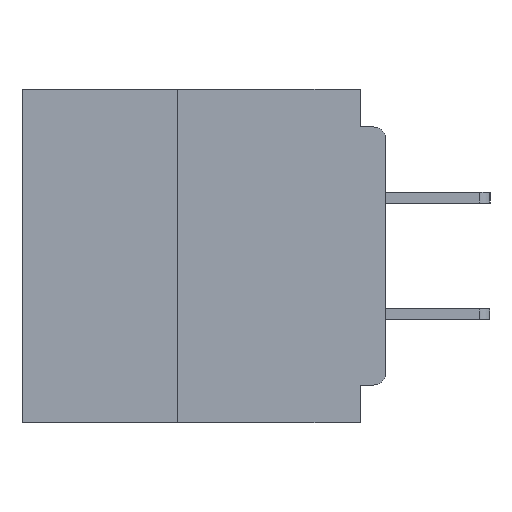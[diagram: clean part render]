
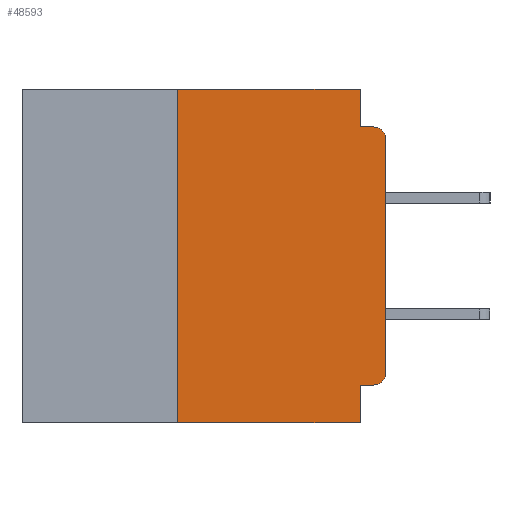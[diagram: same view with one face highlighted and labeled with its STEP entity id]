
A CAD part, left-side view. The second image highlights one B-rep face of the part: STEP entity #48593.
In plain terms, the highlighted planar face has unit normal (-1, 0, 0).
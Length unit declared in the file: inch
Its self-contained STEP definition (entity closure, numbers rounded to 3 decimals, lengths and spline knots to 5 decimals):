
#178 = CARTESIAN_POINT ( 'NONE',  ( 0., 0.031, -0.4 ) ) ;
#2122 = CARTESIAN_POINT ( 'NONE',  ( 0., 0., -0.355 ) ) ;
#2976 = EDGE_CURVE ( 'NONE', #23231, #23133, #15568, .T. ) ;
#4023 = DIRECTION ( 'NONE',  ( 0., 0., -1. ) ) ;
#4742 = CARTESIAN_POINT ( 'NONE',  ( 0., 0.015, -0.355 ) ) ;
#6168 = CARTESIAN_POINT ( 'NONE',  ( 0., 0.031, -0.4 ) ) ;
#6310 = AXIS2_PLACEMENT_3D ( 'NONE', #19619, #46124, #23431 ) ;
#6483 = ORIENTED_EDGE ( 'NONE', *, *, #15444, .F. ) ;
#6874 = DIRECTION ( 'NONE',  ( 0., 0., 1. ) ) ;
#7160 = EDGE_CURVE ( 'NONE', #12666, #23231, #46648, .T. ) ;
#7787 = CARTESIAN_POINT ( 'NONE',  ( 0., 0., -0.045 ) ) ;
#8104 = EDGE_CURVE ( 'NONE', #19189, #9702, #42371, .T. ) ;
#9702 = VERTEX_POINT ( 'NONE', #12455 ) ;
#9875 = LINE ( 'NONE', #178, #12223 ) ;
#12223 = VECTOR ( 'NONE', #4023, 39.37008 ) ;
#12455 = CARTESIAN_POINT ( 'NONE',  ( 0., 0.031, -0.355 ) ) ;
#12594 = DIRECTION ( 'NONE',  ( 0., 0., -1. ) ) ;
#12666 = VERTEX_POINT ( 'NONE', #37422 ) ;
#12769 = EDGE_CURVE ( 'NONE', #9702, #44273, #9875, .T. ) ;
#13081 = VECTOR ( 'NONE', #38442, 39.37008 ) ;
#14164 = ORIENTED_EDGE ( 'NONE', *, *, #8104, .F. ) ;
#14727 = ORIENTED_EDGE ( 'NONE', *, *, #15273, .T. ) ;
#15144 = VECTOR ( 'NONE', #35026, 39.37008 ) ;
#15273 = EDGE_CURVE ( 'NONE', #48046, #44273, #24328, .T. ) ;
#15444 = EDGE_CURVE ( 'NONE', #29797, #28308, #35060, .T. ) ;
#15518 = EDGE_LOOP ( 'NONE', ( #47272, #30776, #42019, #35539, #6483, #49037, #14727, #44966, #14164, #15943 ) ) ;
#15568 = CIRCLE ( 'NONE', #18995, 0.015 ) ;
#15777 = CARTESIAN_POINT ( 'NONE',  ( 0., 0.031, 0. ) ) ;
#15943 = ORIENTED_EDGE ( 'NONE', *, *, #42050, .T. ) ;
#16989 = CARTESIAN_POINT ( 'NONE',  ( 0., 0.25, 0. ) ) ;
#17004 = CARTESIAN_POINT ( 'NONE',  ( 0., 0.015, -0.045 ) ) ;
#17726 = DIRECTION ( 'NONE',  ( 0., 0., -1. ) ) ;
#17768 = DIRECTION ( 'NONE',  ( -1., 0., 0. ) ) ;
#17845 = EDGE_CURVE ( 'NONE', #48046, #29797, #35399, .T. ) ;
#17928 = CARTESIAN_POINT ( 'NONE',  ( 0., 0.015, -0.06 ) ) ;
#18133 = DIRECTION ( 'NONE',  ( 0., 0., -1. ) ) ;
#18995 = AXIS2_PLACEMENT_3D ( 'NONE', #17928, #17768, #17726 ) ;
#19189 = VERTEX_POINT ( 'NONE', #4742 ) ;
#19468 = CARTESIAN_POINT ( 'NONE',  ( 0., 0.437, -0.4 ) ) ;
#19619 = CARTESIAN_POINT ( 'NONE',  ( 0., 0.015, -0.34 ) ) ;
#19837 = VECTOR ( 'NONE', #18133, 39.37008 ) ;
#20613 = DIRECTION ( 'NONE',  ( 0., -1., 0. ) ) ;
#21711 = CARTESIAN_POINT ( 'NONE',  ( 0., 0.031, -0.045 ) ) ;
#22118 = VERTEX_POINT ( 'NONE', #21711 ) ;
#23133 = VERTEX_POINT ( 'NONE', #17004 ) ;
#23231 = VERTEX_POINT ( 'NONE', #40264 ) ;
#23431 = DIRECTION ( 'NONE',  ( 0., 0., -1. ) ) ;
#23543 = CIRCLE ( 'NONE', #6310, 0.015 ) ;
#23827 = PLANE ( 'NONE',  #42882 ) ;
#24328 = LINE ( 'NONE', #19468, #13081 ) ;
#28038 = EDGE_CURVE ( 'NONE', #28308, #22118, #47683, .T. ) ;
#28308 = VERTEX_POINT ( 'NONE', #15777 ) ;
#29552 = CARTESIAN_POINT ( 'NONE',  ( 0., 0., 0. ) ) ;
#29797 = VERTEX_POINT ( 'NONE', #16989 ) ;
#30776 = ORIENTED_EDGE ( 'NONE', *, *, #2976, .T. ) ;
#31210 = CARTESIAN_POINT ( 'NONE',  ( 0., 0.25, -0.4 ) ) ;
#32345 = VECTOR ( 'NONE', #43901, 39.37008 ) ;
#32848 = VECTOR ( 'NONE', #45645, 39.37008 ) ;
#35026 = DIRECTION ( 'NONE',  ( 0., 0., 1. ) ) ;
#35060 = LINE ( 'NONE', #43350, #46237 ) ;
#35348 = DIRECTION ( 'NONE',  ( 1., 0., 0. ) ) ;
#35399 = LINE ( 'NONE', #31210, #15144 ) ;
#35539 = ORIENTED_EDGE ( 'NONE', *, *, #28038, .F. ) ;
#36050 = EDGE_CURVE ( 'NONE', #22118, #23133, #42881, .T. ) ;
#37422 = CARTESIAN_POINT ( 'NONE',  ( 0., 0., -0.34 ) ) ;
#37835 = VECTOR ( 'NONE', #6874, 39.37008 ) ;
#38442 = DIRECTION ( 'NONE',  ( 0., -1., 0. ) ) ;
#40264 = CARTESIAN_POINT ( 'NONE',  ( 0., 0., -0.06 ) ) ;
#42019 = ORIENTED_EDGE ( 'NONE', *, *, #36050, .F. ) ;
#42050 = EDGE_CURVE ( 'NONE', #19189, #12666, #23543, .T. ) ;
#42371 = LINE ( 'NONE', #2122, #32345 ) ;
#42881 = LINE ( 'NONE', #7787, #32848 ) ;
#42882 = AXIS2_PLACEMENT_3D ( 'NONE', #46529, #35348, #12594 ) ;
#43350 = CARTESIAN_POINT ( 'NONE',  ( 0., 0.437, 0. ) ) ;
#43901 = DIRECTION ( 'NONE',  ( 0., 1., 0. ) ) ;
#44273 = VERTEX_POINT ( 'NONE', #6168 ) ;
#44664 = CARTESIAN_POINT ( 'NONE',  ( 0., 0.031, 0. ) ) ;
#44966 = ORIENTED_EDGE ( 'NONE', *, *, #12769, .F. ) ;
#45645 = DIRECTION ( 'NONE',  ( 0., -1., 0. ) ) ;
#45694 = FACE_OUTER_BOUND ( 'NONE', #15518, .T. ) ;
#46124 = DIRECTION ( 'NONE',  ( -1., 0., 0. ) ) ;
#46237 = VECTOR ( 'NONE', #20613, 39.37008 ) ;
#46239 = CARTESIAN_POINT ( 'NONE',  ( 0., 0.25, -0.4 ) ) ;
#46529 = CARTESIAN_POINT ( 'NONE',  ( 0., 0.437, 0. ) ) ;
#46648 = LINE ( 'NONE', #29552, #37835 ) ;
#47272 = ORIENTED_EDGE ( 'NONE', *, *, #7160, .T. ) ;
#47683 = LINE ( 'NONE', #44664, #19837 ) ;
#48046 = VERTEX_POINT ( 'NONE', #46239 ) ;
#48593 = ADVANCED_FACE ( 'NONE', ( #45694 ), #23827, .F. ) ;
#49037 = ORIENTED_EDGE ( 'NONE', *, *, #17845, .F. ) ;
